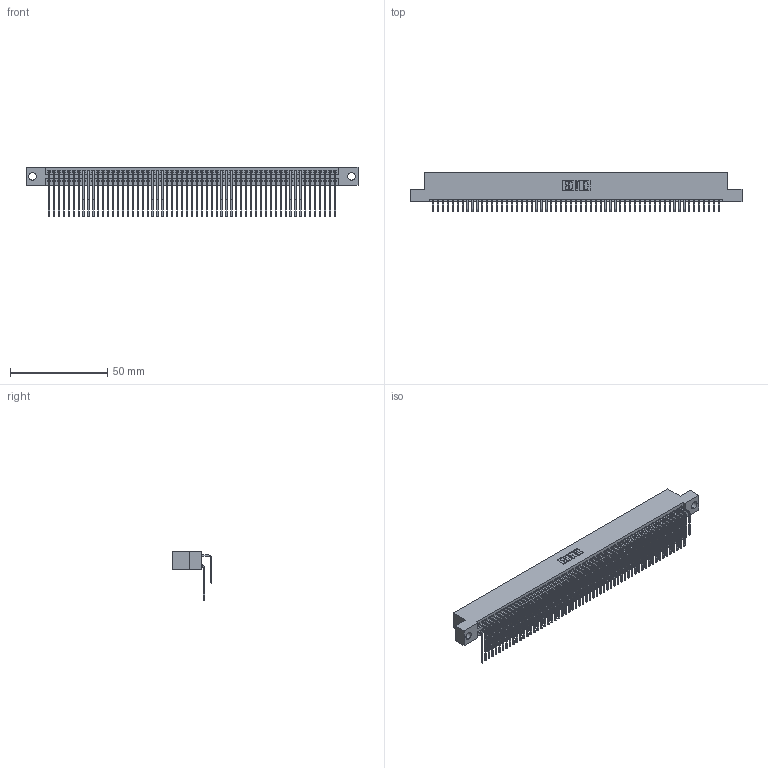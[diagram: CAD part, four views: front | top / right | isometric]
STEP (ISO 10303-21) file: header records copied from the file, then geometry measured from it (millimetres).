
FILE_DESCRIPTION (( 'STEP AP203' ), '1' );
FILE_NAME ('845-118-559-204.STEP', '2018-11-20T23:30:20', ( '' ), ( '' ), 'SwSTEP 2.0', 'SolidWorks 2016', '' );
FILE_SCHEMA (( 'CONFIG_CONTROL_DESIGN' ));
Length unit declared in the file: inch
Products named in the file (4): 845 Part_Flush Mounting Lugs - 0.156 Dia-TH; 345-292-001_558 559 Tail - 1; 345-292-001_559 Tail - 2; 845-118-559-204
Assembly tree (119 placements, depth 2):
  845-118-559-204
    845 Part_Flush Mounting Lugs - 0.156 Dia-TH
    345-292-001_558 559 Tail - 1  x59
    345-292-001_559 Tail - 2  x59
Bounding box: 171.07 x 20.56 x 25.53 mm (x, y, z)
Volume: 17368.5 mm3; surface area: 29018.9 mm2
Topology: 119 solids, 119 shells, 6262 faces, 18631 edges, 12262 vertices
Faces by surface type: plane 4210, cylinder 2052
Entity records: 45659 total; most frequent: CARTESIAN_POINT 7683, ORIENTED_EDGE 7566, DIRECTION 6727, EDGE_CURVE 3783, LINE 3375, VECTOR 3375, VERTEX_POINT 2518, AXIS2_PLACEMENT_3D 1676
